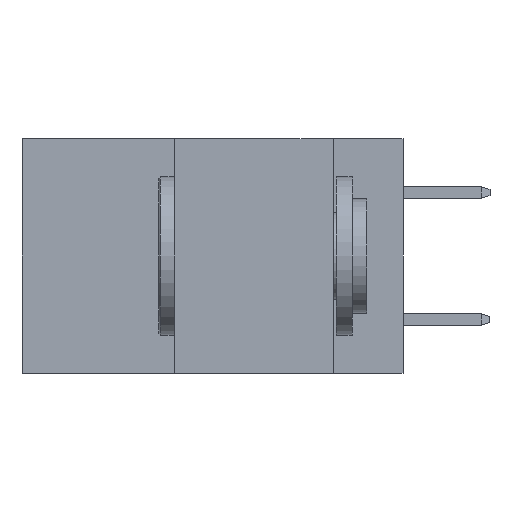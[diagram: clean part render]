
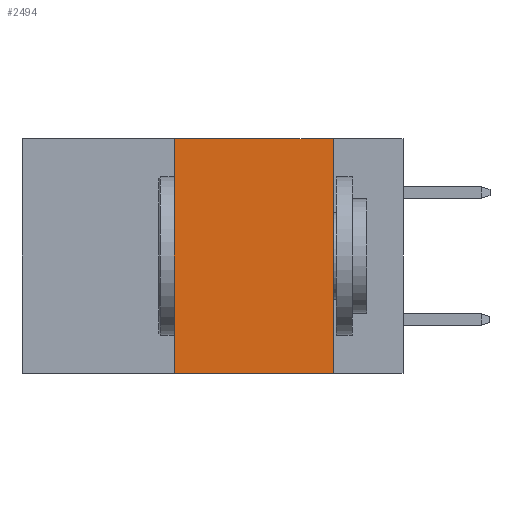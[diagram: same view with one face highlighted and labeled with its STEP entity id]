
A CAD part, left-side view. The second image highlights one B-rep face of the part: STEP entity #2494.
In plain terms, the highlighted planar face has unit normal (-1, 0, 0).
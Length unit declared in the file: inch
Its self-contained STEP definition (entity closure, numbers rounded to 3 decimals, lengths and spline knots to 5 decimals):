
#588 = FACE_OUTER_BOUND ( 'NONE', #968, .T. ) ;
#620 = VERTEX_POINT ( 'NONE', #7616 ) ;
#968 = EDGE_LOOP ( 'NONE', ( #12371, #7096, #6884, #9259 ) ) ;
#1287 = DIRECTION ( 'NONE',  ( 0., 0., 1. ) ) ;
#1938 = EDGE_CURVE ( 'NONE', #2469, #5572, #11324, .T. ) ;
#2023 = AXIS2_PLACEMENT_3D ( 'NONE', #7172, #2406, #11729 ) ;
#2406 = DIRECTION ( 'NONE',  ( 1., 0., 0. ) ) ;
#2469 = VERTEX_POINT ( 'NONE', #7114 ) ;
#2494 = ADVANCED_FACE ( 'NONE', ( #588 ), #4419, .F. ) ;
#3956 = DIRECTION ( 'NONE',  ( 0., 0., -1. ) ) ;
#4419 = PLANE ( 'NONE',  #2023 ) ;
#4647 = VECTOR ( 'NONE', #1287, 39.37008 ) ;
#5502 = DIRECTION ( 'NONE',  ( 0., -1., 0. ) ) ;
#5572 = VERTEX_POINT ( 'NONE', #8511 ) ;
#5764 = CARTESIAN_POINT ( 'NONE',  ( 0., 0.6, 0. ) ) ;
#6884 = ORIENTED_EDGE ( 'NONE', *, *, #10606, .F. ) ;
#6988 = CARTESIAN_POINT ( 'NONE',  ( 0., 0.36, 0. ) ) ;
#7016 = CARTESIAN_POINT ( 'NONE',  ( 0., 0.36, -0.37 ) ) ;
#7096 = ORIENTED_EDGE ( 'NONE', *, *, #11733, .F. ) ;
#7114 = CARTESIAN_POINT ( 'NONE',  ( 0., 0.11, 0. ) ) ;
#7121 = LINE ( 'NONE', #6988, #4647 ) ;
#7172 = CARTESIAN_POINT ( 'NONE',  ( 0., 0.6, 0. ) ) ;
#7550 = CARTESIAN_POINT ( 'NONE',  ( 0., 0.6, -0.37 ) ) ;
#7571 = CARTESIAN_POINT ( 'NONE',  ( 0., 0.11, 0. ) ) ;
#7616 = CARTESIAN_POINT ( 'NONE',  ( 0., 0.36, 0. ) ) ;
#7827 = VECTOR ( 'NONE', #11276, 39.37008 ) ;
#8455 = VERTEX_POINT ( 'NONE', #7016 ) ;
#8511 = CARTESIAN_POINT ( 'NONE',  ( 0., 0.11, -0.37 ) ) ;
#9259 = ORIENTED_EDGE ( 'NONE', *, *, #10284, .T. ) ;
#9750 = VECTOR ( 'NONE', #5502, 39.37008 ) ;
#10248 = LINE ( 'NONE', #7550, #9750 ) ;
#10284 = EDGE_CURVE ( 'NONE', #8455, #5572, #10248, .T. ) ;
#10528 = LINE ( 'NONE', #5764, #7827 ) ;
#10606 = EDGE_CURVE ( 'NONE', #8455, #620, #7121, .T. ) ;
#11276 = DIRECTION ( 'NONE',  ( 0., -1., 0. ) ) ;
#11324 = LINE ( 'NONE', #7571, #11963 ) ;
#11729 = DIRECTION ( 'NONE',  ( 0., 0., -1. ) ) ;
#11733 = EDGE_CURVE ( 'NONE', #620, #2469, #10528, .T. ) ;
#11963 = VECTOR ( 'NONE', #3956, 39.37008 ) ;
#12371 = ORIENTED_EDGE ( 'NONE', *, *, #1938, .F. ) ;
